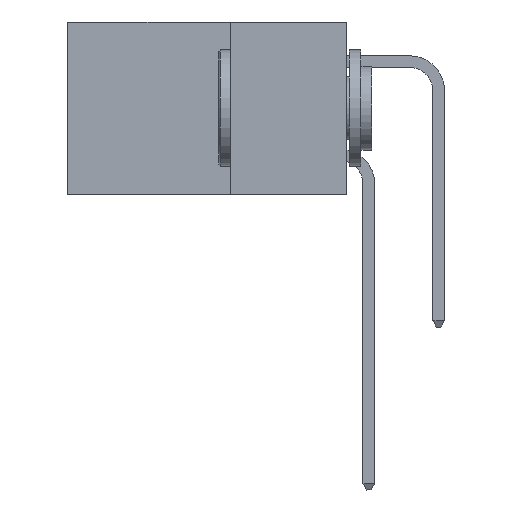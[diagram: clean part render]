
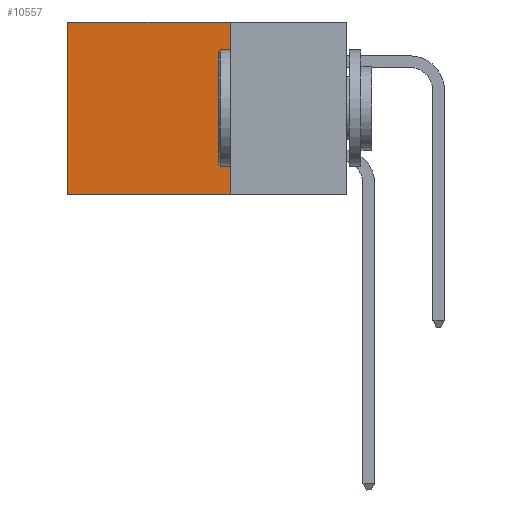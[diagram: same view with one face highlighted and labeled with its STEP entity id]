
A CAD part, left-side view. The second image highlights one B-rep face of the part: STEP entity #10557.
In plain terms, the highlighted planar face has unit normal (-1, 0, 0).
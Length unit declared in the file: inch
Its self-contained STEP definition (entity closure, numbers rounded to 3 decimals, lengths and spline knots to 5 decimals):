
#111 = LINE ( 'NONE', #14620, #13810 ) ;
#570 = CARTESIAN_POINT ( 'NONE',  ( 0.2875, 0.6, 0. ) ) ;
#948 = CARTESIAN_POINT ( 'NONE',  ( 0.2875, 0.25, 0. ) ) ;
#1289 = VERTEX_POINT ( 'NONE', #3597 ) ;
#1554 = EDGE_LOOP ( 'NONE', ( #7129, #15327, #6235, #8736 ) ) ;
#2188 = EDGE_CURVE ( 'NONE', #11210, #16524, #11465, .T. ) ;
#2506 = DIRECTION ( 'NONE',  ( 0., 0., -1. ) ) ;
#3099 = EDGE_CURVE ( 'NONE', #6983, #11210, #5231, .T. ) ;
#3211 = CARTESIAN_POINT ( 'NONE',  ( 0.2875, 0.25, -0.37 ) ) ;
#3597 = CARTESIAN_POINT ( 'NONE',  ( 0.2875, 0.25, -0.37 ) ) ;
#3963 = LINE ( 'NONE', #3211, #10546 ) ;
#4682 = CARTESIAN_POINT ( 'NONE',  ( 0.2875, 0.6, 0. ) ) ;
#5231 = LINE ( 'NONE', #12459, #15364 ) ;
#6235 = ORIENTED_EDGE ( 'NONE', *, *, #10905, .F. ) ;
#6983 = VERTEX_POINT ( 'NONE', #948 ) ;
#6986 = DIRECTION ( 'NONE',  ( 1., 0., 0. ) ) ;
#7129 = ORIENTED_EDGE ( 'NONE', *, *, #2188, .T. ) ;
#8345 = VECTOR ( 'NONE', #2506, 39.37008 ) ;
#8736 = ORIENTED_EDGE ( 'NONE', *, *, #3099, .T. ) ;
#8890 = AXIS2_PLACEMENT_3D ( 'NONE', #10934, #6986, #16189 ) ;
#9808 = DIRECTION ( 'NONE',  ( 0., 1., 0. ) ) ;
#10546 = VECTOR ( 'NONE', #9808, 39.37008 ) ;
#10557 = ADVANCED_FACE ( 'NONE', ( #16857 ), #14914, .F. ) ;
#10905 = EDGE_CURVE ( 'NONE', #6983, #1289, #111, .T. ) ;
#10934 = CARTESIAN_POINT ( 'NONE',  ( 0.2875, 0.25, 0. ) ) ;
#11210 = VERTEX_POINT ( 'NONE', #4682 ) ;
#11465 = LINE ( 'NONE', #570, #8345 ) ;
#11489 = CARTESIAN_POINT ( 'NONE',  ( 0.2875, 0.6, -0.37 ) ) ;
#11802 = EDGE_CURVE ( 'NONE', #1289, #16524, #3963, .T. ) ;
#12382 = DIRECTION ( 'NONE',  ( 0., 1., 0. ) ) ;
#12459 = CARTESIAN_POINT ( 'NONE',  ( 0.2875, 0.25, 0. ) ) ;
#13810 = VECTOR ( 'NONE', #15861, 39.37008 ) ;
#14620 = CARTESIAN_POINT ( 'NONE',  ( 0.2875, 0.25, 0. ) ) ;
#14914 = PLANE ( 'NONE',  #8890 ) ;
#15327 = ORIENTED_EDGE ( 'NONE', *, *, #11802, .F. ) ;
#15364 = VECTOR ( 'NONE', #12382, 39.37008 ) ;
#15861 = DIRECTION ( 'NONE',  ( 0., 0., -1. ) ) ;
#16189 = DIRECTION ( 'NONE',  ( 0., 0., -1. ) ) ;
#16524 = VERTEX_POINT ( 'NONE', #11489 ) ;
#16857 = FACE_OUTER_BOUND ( 'NONE', #1554, .T. ) ;
